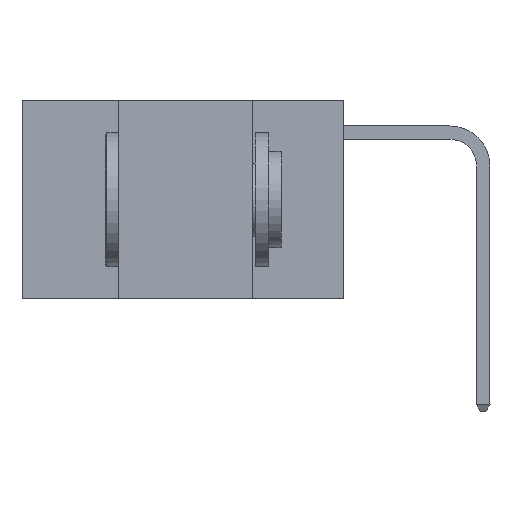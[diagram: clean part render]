
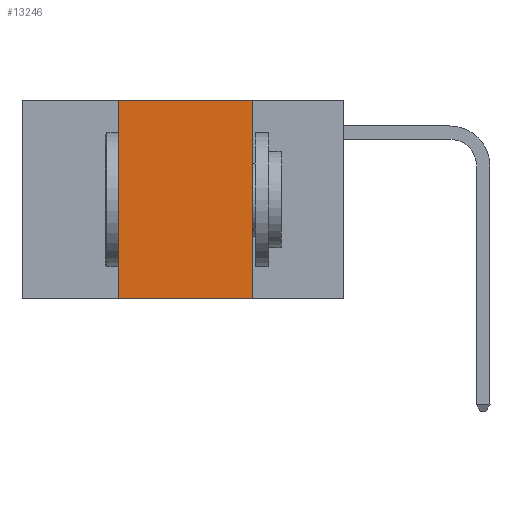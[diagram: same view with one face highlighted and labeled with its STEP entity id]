
A CAD part, left-side view. The second image highlights one B-rep face of the part: STEP entity #13246.
In plain terms, the highlighted planar face has unit normal (-1, 0, 0).
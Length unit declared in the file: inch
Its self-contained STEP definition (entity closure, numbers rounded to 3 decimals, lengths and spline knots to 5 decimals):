
#28 = VECTOR ( 'NONE', #13688, 39.37008 ) ;
#228 = VECTOR ( 'NONE', #14882, 39.37008 ) ;
#379 = AXIS2_PLACEMENT_3D ( 'NONE', #8979, #1829, #10210 ) ;
#775 = EDGE_CURVE ( 'NONE', #11587, #6503, #4450, .T. ) ;
#1783 = PLANE ( 'NONE',  #379 ) ;
#1793 = CARTESIAN_POINT ( 'NONE',  ( 0., 0.42, 0. ) ) ;
#1829 = DIRECTION ( 'NONE',  ( 1., 0., 0. ) ) ;
#3028 = DIRECTION ( 'NONE',  ( 0., 0., 1. ) ) ;
#3333 = CARTESIAN_POINT ( 'NONE',  ( 0., 0.42, 0. ) ) ;
#4220 = CARTESIAN_POINT ( 'NONE',  ( 0., 0.6, -0.37 ) ) ;
#4364 = CARTESIAN_POINT ( 'NONE',  ( 0., 0.42, -0.37 ) ) ;
#4450 = LINE ( 'NONE', #1793, #7299 ) ;
#6009 = VECTOR ( 'NONE', #7415, 39.37008 ) ;
#6237 = CARTESIAN_POINT ( 'NONE',  ( 0., 0.6, 0. ) ) ;
#6420 = LINE ( 'NONE', #4220, #28 ) ;
#6503 = VERTEX_POINT ( 'NONE', #3333 ) ;
#6617 = LINE ( 'NONE', #7922, #228 ) ;
#7150 = CARTESIAN_POINT ( 'NONE',  ( 0., 0.17, 0. ) ) ;
#7299 = VECTOR ( 'NONE', #3028, 39.37008 ) ;
#7415 = DIRECTION ( 'NONE',  ( 0., -1., 0. ) ) ;
#7906 = EDGE_CURVE ( 'NONE', #6503, #8405, #9905, .T. ) ;
#7922 = CARTESIAN_POINT ( 'NONE',  ( 0., 0.17, 0. ) ) ;
#8066 = ORIENTED_EDGE ( 'NONE', *, *, #15290, .F. ) ;
#8284 = ORIENTED_EDGE ( 'NONE', *, *, #7906, .F. ) ;
#8405 = VERTEX_POINT ( 'NONE', #7150 ) ;
#8915 = ORIENTED_EDGE ( 'NONE', *, *, #775, .F. ) ;
#8962 = ORIENTED_EDGE ( 'NONE', *, *, #11493, .T. ) ;
#8979 = CARTESIAN_POINT ( 'NONE',  ( 0., 0.6, 0. ) ) ;
#9905 = LINE ( 'NONE', #6237, #6009 ) ;
#9926 = EDGE_LOOP ( 'NONE', ( #8066, #8284, #8915, #8962 ) ) ;
#10210 = DIRECTION ( 'NONE',  ( 0., 0., -1. ) ) ;
#11429 = VERTEX_POINT ( 'NONE', #12468 ) ;
#11493 = EDGE_CURVE ( 'NONE', #11587, #11429, #6420, .T. ) ;
#11587 = VERTEX_POINT ( 'NONE', #4364 ) ;
#12468 = CARTESIAN_POINT ( 'NONE',  ( 0., 0.17, -0.37 ) ) ;
#13246 = ADVANCED_FACE ( 'NONE', ( #14918 ), #1783, .F. ) ;
#13688 = DIRECTION ( 'NONE',  ( 0., -1., 0. ) ) ;
#14882 = DIRECTION ( 'NONE',  ( 0., 0., -1. ) ) ;
#14918 = FACE_OUTER_BOUND ( 'NONE', #9926, .T. ) ;
#15290 = EDGE_CURVE ( 'NONE', #8405, #11429, #6617, .T. ) ;
